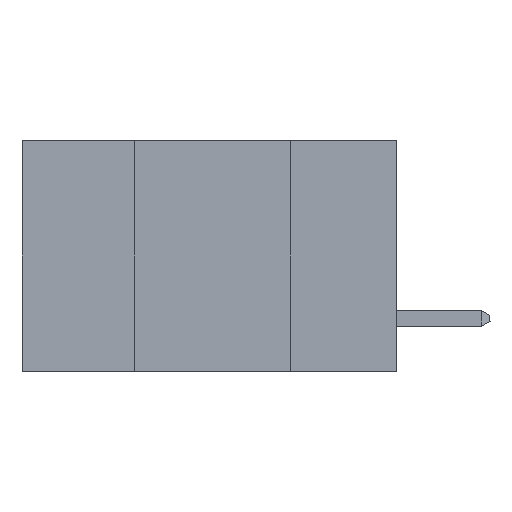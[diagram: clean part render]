
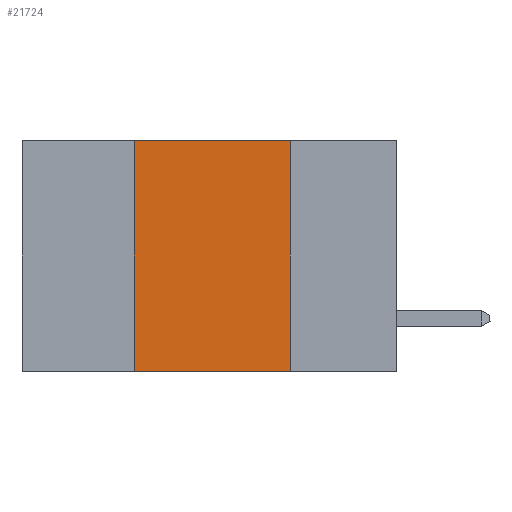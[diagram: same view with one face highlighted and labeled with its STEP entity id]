
A CAD part, left-side view. The second image highlights one B-rep face of the part: STEP entity #21724.
In plain terms, the highlighted planar face has unit normal (-1, 0, 0).
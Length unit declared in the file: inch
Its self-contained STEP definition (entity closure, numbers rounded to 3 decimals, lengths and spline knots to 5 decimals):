
#26 = CARTESIAN_POINT ( 'NONE',  ( 0., 0.42, 0. ) ) ;
#1509 = EDGE_CURVE ( 'NONE', #4102, #2309, #7830, .T. ) ;
#1952 = EDGE_CURVE ( 'NONE', #12367, #17439, #4846, .T. ) ;
#2309 = VERTEX_POINT ( 'NONE', #17570 ) ;
#2476 = CARTESIAN_POINT ( 'NONE',  ( 0., 0.6, 0. ) ) ;
#2527 = ORIENTED_EDGE ( 'NONE', *, *, #1952, .F. ) ;
#3253 = EDGE_CURVE ( 'NONE', #12367, #2309, #20872, .T. ) ;
#3439 = CARTESIAN_POINT ( 'NONE',  ( 0., 0.17, 0. ) ) ;
#3994 = CARTESIAN_POINT ( 'NONE',  ( 0., 0.42, 0. ) ) ;
#4102 = VERTEX_POINT ( 'NONE', #5017 ) ;
#4846 = LINE ( 'NONE', #26, #18251 ) ;
#5017 = CARTESIAN_POINT ( 'NONE',  ( 0., 0.17, 0. ) ) ;
#5043 = DIRECTION ( 'NONE',  ( 0., -1., 0. ) ) ;
#5906 = VECTOR ( 'NONE', #5043, 39.37008 ) ;
#5987 = VECTOR ( 'NONE', #22193, 39.37008 ) ;
#6441 = PLANE ( 'NONE',  #8937 ) ;
#7103 = DIRECTION ( 'NONE',  ( 0., 0., -1. ) ) ;
#7830 = LINE ( 'NONE', #3439, #12003 ) ;
#8094 = EDGE_CURVE ( 'NONE', #17439, #4102, #18698, .T. ) ;
#8162 = ORIENTED_EDGE ( 'NONE', *, *, #1509, .F. ) ;
#8426 = ORIENTED_EDGE ( 'NONE', *, *, #3253, .T. ) ;
#8937 = AXIS2_PLACEMENT_3D ( 'NONE', #13913, #21662, #10323 ) ;
#10323 = DIRECTION ( 'NONE',  ( 0., 0., -1. ) ) ;
#11009 = FACE_OUTER_BOUND ( 'NONE', #21879, .T. ) ;
#12003 = VECTOR ( 'NONE', #7103, 39.37008 ) ;
#12367 = VERTEX_POINT ( 'NONE', #22691 ) ;
#12795 = CARTESIAN_POINT ( 'NONE',  ( 0., 0.6, -0.37 ) ) ;
#13913 = CARTESIAN_POINT ( 'NONE',  ( 0., 0.6, 0. ) ) ;
#17439 = VERTEX_POINT ( 'NONE', #3994 ) ;
#17570 = CARTESIAN_POINT ( 'NONE',  ( 0., 0.17, -0.37 ) ) ;
#18251 = VECTOR ( 'NONE', #18962, 39.37008 ) ;
#18698 = LINE ( 'NONE', #2476, #5906 ) ;
#18934 = ORIENTED_EDGE ( 'NONE', *, *, #8094, .F. ) ;
#18962 = DIRECTION ( 'NONE',  ( 0., 0., 1. ) ) ;
#20872 = LINE ( 'NONE', #12795, #5987 ) ;
#21662 = DIRECTION ( 'NONE',  ( 1., 0., 0. ) ) ;
#21724 = ADVANCED_FACE ( 'NONE', ( #11009 ), #6441, .F. ) ;
#21879 = EDGE_LOOP ( 'NONE', ( #8162, #18934, #2527, #8426 ) ) ;
#22193 = DIRECTION ( 'NONE',  ( 0., -1., 0. ) ) ;
#22691 = CARTESIAN_POINT ( 'NONE',  ( 0., 0.42, -0.37 ) ) ;
